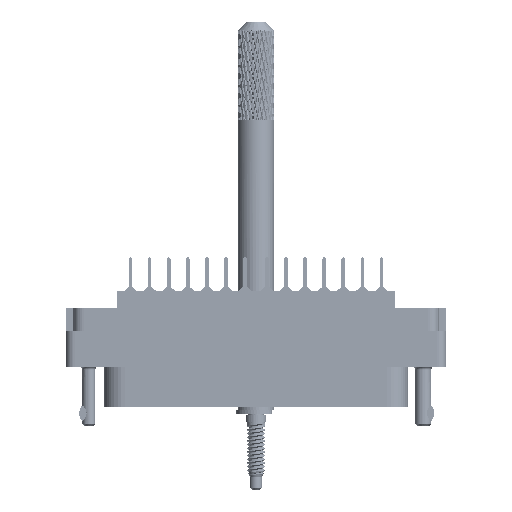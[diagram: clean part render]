
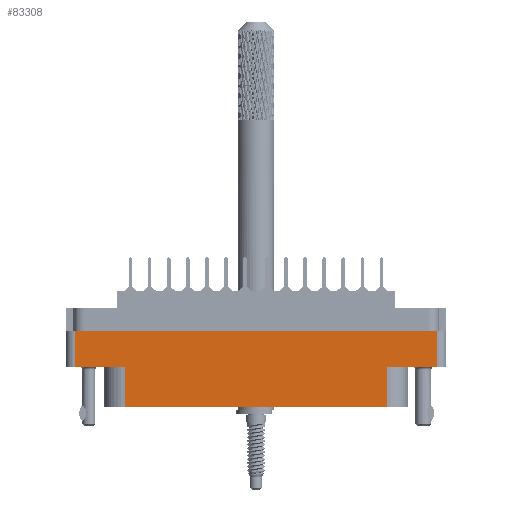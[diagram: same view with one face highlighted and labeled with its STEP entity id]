
A CAD part, front view. The second image highlights one B-rep face of the part: STEP entity #83308.
In plain terms, the highlighted planar face has unit normal (0, -1, 0).
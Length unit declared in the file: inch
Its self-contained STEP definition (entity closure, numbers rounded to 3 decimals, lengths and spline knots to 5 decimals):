
#1589 = VERTEX_POINT ( 'NONE', #84403 ) ;
#2091 = LINE ( 'NONE', #104745, #123779 ) ;
#4062 = VERTEX_POINT ( 'NONE', #12918 ) ;
#4214 = LINE ( 'NONE', #38279, #37162 ) ;
#5220 = LINE ( 'NONE', #112709, #20257 ) ;
#6753 = ORIENTED_EDGE ( 'NONE', *, *, #114503, .F. ) ;
#7979 = LINE ( 'NONE', #18884, #42542 ) ;
#12333 = LINE ( 'NONE', #56949, #70881 ) ;
#12634 = ORIENTED_EDGE ( 'NONE', *, *, #47024, .T. ) ;
#12918 = CARTESIAN_POINT ( 'NONE',  ( 0.895, -0.438, -0.52 ) ) ;
#13705 = EDGE_CURVE ( 'NONE', #71289, #26214, #7979, .T. ) ;
#15660 = CARTESIAN_POINT ( 'NONE',  ( 1.2335, -0.438, -0.52 ) ) ;
#18884 = CARTESIAN_POINT ( 'NONE',  ( 1.2335, -0.438, -0.789 ) ) ;
#18927 = VERTEX_POINT ( 'NONE', #102508 ) ;
#20257 = VECTOR ( 'NONE', #64832, 39.37008 ) ;
#26214 = VERTEX_POINT ( 'NONE', #62580 ) ;
#29677 = DIRECTION ( 'NONE',  ( -1., 0., 0. ) ) ;
#34850 = VERTEX_POINT ( 'NONE', #112667 ) ;
#36745 = DIRECTION ( 'NONE',  ( -1., 0., 0. ) ) ;
#37162 = VECTOR ( 'NONE', #95845, 39.37008 ) ;
#37175 = DIRECTION ( 'NONE',  ( 1., 0., 0. ) ) ;
#38279 = CARTESIAN_POINT ( 'NONE',  ( -1.2335, -0.438, -0.789 ) ) ;
#42542 = VECTOR ( 'NONE', #55423, 39.37008 ) ;
#43001 = DIRECTION ( 'NONE',  ( 0., -1., 0. ) ) ;
#44220 = VECTOR ( 'NONE', #109496, 39.37008 ) ;
#47024 = EDGE_CURVE ( 'NONE', #18927, #34850, #4214, .T. ) ;
#48493 = ORIENTED_EDGE ( 'NONE', *, *, #55279, .F. ) ;
#52275 = EDGE_CURVE ( 'NONE', #79031, #98214, #106228, .T. ) ;
#54301 = PLANE ( 'NONE',  #85427 ) ;
#54990 = EDGE_CURVE ( 'NONE', #98214, #4062, #5220, .T. ) ;
#55279 = EDGE_CURVE ( 'NONE', #18927, #26214, #119424, .T. ) ;
#55423 = DIRECTION ( 'NONE',  ( 0., 0., 1. ) ) ;
#56949 = CARTESIAN_POINT ( 'NONE',  ( -0.895, -0.438, -0.789 ) ) ;
#62580 = CARTESIAN_POINT ( 'NONE',  ( 1.2335, -0.438, -0.274 ) ) ;
#63536 = CARTESIAN_POINT ( 'NONE',  ( -1.2955, -0.438, -0.789 ) ) ;
#64832 = DIRECTION ( 'NONE',  ( 0., 0., 1. ) ) ;
#65731 = CARTESIAN_POINT ( 'NONE',  ( -1.2955, -0.438, -0.789 ) ) ;
#70881 = VECTOR ( 'NONE', #122485, 39.37008 ) ;
#71289 = VERTEX_POINT ( 'NONE', #15660 ) ;
#76742 = CARTESIAN_POINT ( 'NONE',  ( 0., -0.438, -0.52 ) ) ;
#77623 = FACE_OUTER_BOUND ( 'NONE', #112124, .T. ) ;
#78275 = ORIENTED_EDGE ( 'NONE', *, *, #97637, .F. ) ;
#79031 = VERTEX_POINT ( 'NONE', #86870 ) ;
#79311 = VECTOR ( 'NONE', #37175, 39.37008 ) ;
#83308 = ADVANCED_FACE ( 'NONE', ( #77623 ), #54301, .T. ) ;
#84403 = CARTESIAN_POINT ( 'NONE',  ( -0.895, -0.438, -0.52 ) ) ;
#85427 = AXIS2_PLACEMENT_3D ( 'NONE', #63536, #43001, #110173 ) ;
#86870 = CARTESIAN_POINT ( 'NONE',  ( -0.895, -0.438, -0.789 ) ) ;
#88330 = CARTESIAN_POINT ( 'NONE',  ( 0.895, -0.438, -0.789 ) ) ;
#89398 = CARTESIAN_POINT ( 'NONE',  ( 0., -0.438, -0.274 ) ) ;
#89412 = VECTOR ( 'NONE', #29677, 39.37008 ) ;
#95845 = DIRECTION ( 'NONE',  ( 0., 0., -1. ) ) ;
#97637 = EDGE_CURVE ( 'NONE', #71289, #4062, #114894, .T. ) ;
#98214 = VERTEX_POINT ( 'NONE', #88330 ) ;
#100127 = EDGE_CURVE ( 'NONE', #1589, #79031, #12333, .T. ) ;
#102508 = CARTESIAN_POINT ( 'NONE',  ( -1.2335, -0.438, -0.274 ) ) ;
#104745 = CARTESIAN_POINT ( 'NONE',  ( 0., -0.438, -0.52 ) ) ;
#105213 = ORIENTED_EDGE ( 'NONE', *, *, #54990, .T. ) ;
#106022 = ORIENTED_EDGE ( 'NONE', *, *, #52275, .T. ) ;
#106228 = LINE ( 'NONE', #65731, #79311 ) ;
#109496 = DIRECTION ( 'NONE',  ( 1., 0., 0. ) ) ;
#110173 = DIRECTION ( 'NONE',  ( 0., 0., -1. ) ) ;
#112124 = EDGE_LOOP ( 'NONE', ( #48493, #12634, #6753, #112751, #106022, #105213, #78275, #121810 ) ) ;
#112667 = CARTESIAN_POINT ( 'NONE',  ( -1.2335, -0.438, -0.52 ) ) ;
#112709 = CARTESIAN_POINT ( 'NONE',  ( 0.895, -0.438, -0.52 ) ) ;
#112751 = ORIENTED_EDGE ( 'NONE', *, *, #100127, .T. ) ;
#114503 = EDGE_CURVE ( 'NONE', #1589, #34850, #2091, .T. ) ;
#114894 = LINE ( 'NONE', #76742, #89412 ) ;
#119424 = LINE ( 'NONE', #89398, #44220 ) ;
#121810 = ORIENTED_EDGE ( 'NONE', *, *, #13705, .T. ) ;
#122485 = DIRECTION ( 'NONE',  ( 0., 0., -1. ) ) ;
#123779 = VECTOR ( 'NONE', #36745, 39.37008 ) ;
